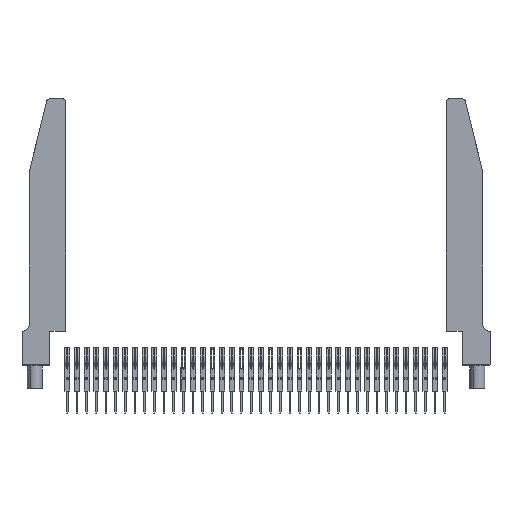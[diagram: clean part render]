
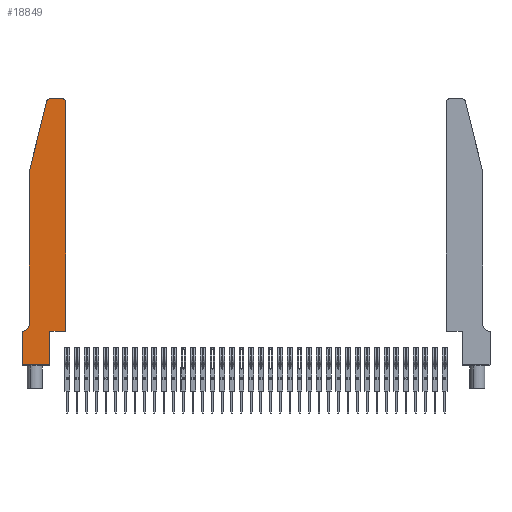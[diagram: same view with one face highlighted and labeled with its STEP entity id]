
A CAD part, top view. The second image highlights one B-rep face of the part: STEP entity #18849.
In plain terms, the highlighted planar face has unit normal (0, 0, 1).
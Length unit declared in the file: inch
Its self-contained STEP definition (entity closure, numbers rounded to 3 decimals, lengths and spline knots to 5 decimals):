
#72 = EDGE_CURVE ( 'NONE', #14185, #10593, #6628, .T. ) ;
#424 = ORIENTED_EDGE ( 'NONE', *, *, #72, .T. ) ;
#1006 = ORIENTED_EDGE ( 'NONE', *, *, #3949, .T. ) ;
#2183 = EDGE_CURVE ( 'NONE', #3761, #11347, #15558, .T. ) ;
#2339 = FACE_OUTER_BOUND ( 'NONE', #12901, .T. ) ;
#3177 = DIRECTION ( 'NONE',  ( -1., 0., 0. ) ) ;
#3275 = CARTESIAN_POINT ( 'NONE',  ( 0.2605, 2.75, 0.37 ) ) ;
#3415 = ORIENTED_EDGE ( 'NONE', *, *, #25045, .T. ) ;
#3742 = ORIENTED_EDGE ( 'NONE', *, *, #20649, .T. ) ;
#3761 = VERTEX_POINT ( 'NONE', #29488 ) ;
#3949 = EDGE_CURVE ( 'NONE', #28144, #14464, #5314, .T. ) ;
#4576 = VERTEX_POINT ( 'NONE', #20757 ) ;
#5207 = DIRECTION ( 'NONE',  ( -1., 0., 0. ) ) ;
#5306 = CARTESIAN_POINT ( 'NONE',  ( 0.2865, 0.35, 0.37 ) ) ;
#5314 = CIRCLE ( 'NONE', #13346, 0.07 ) ;
#5573 = VERTEX_POINT ( 'NONE', #18539 ) ;
#5587 = DIRECTION ( 'NONE',  ( -1., 0., 0. ) ) ;
#6424 = VECTOR ( 'NONE', #5587, 39.37008 ) ;
#6628 = LINE ( 'NONE', #18427, #9230 ) ;
#7030 = LINE ( 'NONE', #23628, #14231 ) ;
#7182 = VERTEX_POINT ( 'NONE', #7371 ) ;
#7371 = CARTESIAN_POINT ( 'NONE',  ( 0.25487, 2.72718, 0.37 ) ) ;
#7694 = DIRECTION ( 'NONE',  ( 0., 1., 0. ) ) ;
#8362 = CARTESIAN_POINT ( 'NONE',  ( 0.0055, 0.42, 0.37 ) ) ;
#8499 = DIRECTION ( 'NONE',  ( 0., -1., 0. ) ) ;
#8821 = CIRCLE ( 'NONE', #21907, 0.03 ) ;
#9230 = VECTOR ( 'NONE', #7694, 39.37008 ) ;
#9520 = VECTOR ( 'NONE', #32778, 39.37008 ) ;
#9580 = CARTESIAN_POINT ( 'NONE',  ( 0., 0.35, 0.37 ) ) ;
#10593 = VERTEX_POINT ( 'NONE', #5306 ) ;
#10608 = CARTESIAN_POINT ( 'NONE',  ( 0.4205, 2.75, 0.37 ) ) ;
#10736 = CARTESIAN_POINT ( 'NONE',  ( 0., 0.35, 0.37 ) ) ;
#10897 = ORIENTED_EDGE ( 'NONE', *, *, #23701, .T. ) ;
#11187 = EDGE_CURVE ( 'NONE', #7182, #29324, #7030, .T. ) ;
#11347 = VERTEX_POINT ( 'NONE', #10608 ) ;
#12293 = LINE ( 'NONE', #17648, #28172 ) ;
#12449 = VECTOR ( 'NONE', #31641, 39.37008 ) ;
#12901 = EDGE_LOOP ( 'NONE', ( #17440, #3742, #28590, #15875, #1006, #10897, #27812, #3415, #424, #24898, #13096, #30906 ) ) ;
#13096 = ORIENTED_EDGE ( 'NONE', *, *, #25732, .T. ) ;
#13346 = AXIS2_PLACEMENT_3D ( 'NONE', #8362, #14113, #3177 ) ;
#13997 = CARTESIAN_POINT ( 'NONE',  ( 0., 0., 0.37 ) ) ;
#14113 = DIRECTION ( 'NONE',  ( 0., 0., -1. ) ) ;
#14185 = VERTEX_POINT ( 'NONE', #18799 ) ;
#14231 = VECTOR ( 'NONE', #17410, 39.37008 ) ;
#14241 = VERTEX_POINT ( 'NONE', #21277 ) ;
#14464 = VERTEX_POINT ( 'NONE', #22531 ) ;
#15558 = CIRCLE ( 'NONE', #31065, 0.03 ) ;
#15684 = DIRECTION ( 'NONE',  ( 0., 0., 1. ) ) ;
#15696 = LINE ( 'NONE', #15880, #34674 ) ;
#15875 = ORIENTED_EDGE ( 'NONE', *, *, #19548, .T. ) ;
#15880 = CARTESIAN_POINT ( 'NONE',  ( 0.4505, 0.35, 0.37 ) ) ;
#16834 = LINE ( 'NONE', #13997, #9520 ) ;
#17410 = DIRECTION ( 'NONE',  ( -0.239, -0.971, 0. ) ) ;
#17440 = ORIENTED_EDGE ( 'NONE', *, *, #27198, .T. ) ;
#17648 = CARTESIAN_POINT ( 'NONE',  ( 0.0755, 2., 0.37 ) ) ;
#18427 = CARTESIAN_POINT ( 'NONE',  ( 0.2865, 0.35, 0.37 ) ) ;
#18539 = CARTESIAN_POINT ( 'NONE',  ( 0.284, 2.75, 0.37 ) ) ;
#18799 = CARTESIAN_POINT ( 'NONE',  ( 0.2865, 0., 0.37 ) ) ;
#18849 = ADVANCED_FACE ( 'NONE', ( #2339 ), #35235, .T. ) ;
#19548 = EDGE_CURVE ( 'NONE', #29324, #28144, #12293, .T. ) ;
#19966 = CARTESIAN_POINT ( 'NONE',  ( 0.4205, 2.72, 0.37 ) ) ;
#20649 = EDGE_CURVE ( 'NONE', #5573, #7182, #8821, .T. ) ;
#20757 = CARTESIAN_POINT ( 'NONE',  ( 0., 0., 0.37 ) ) ;
#21118 = LINE ( 'NONE', #29556, #29458 ) ;
#21277 = CARTESIAN_POINT ( 'NONE',  ( 0.4505, 0.35, 0.37 ) ) ;
#21907 = AXIS2_PLACEMENT_3D ( 'NONE', #23146, #15684, #34471 ) ;
#22531 = CARTESIAN_POINT ( 'NONE',  ( 0.0055, 0.35, 0.37 ) ) ;
#22934 = LINE ( 'NONE', #33198, #24058 ) ;
#23146 = CARTESIAN_POINT ( 'NONE',  ( 0.284, 2.72, 0.37 ) ) ;
#23316 = DIRECTION ( 'NONE',  ( 1., 0., 0. ) ) ;
#23628 = CARTESIAN_POINT ( 'NONE',  ( 0.0755, 2., 0.37 ) ) ;
#23701 = EDGE_CURVE ( 'NONE', #14464, #28133, #21118, .T. ) ;
#24058 = VECTOR ( 'NONE', #8499, 39.37008 ) ;
#24898 = ORIENTED_EDGE ( 'NONE', *, *, #33653, .T. ) ;
#25045 = EDGE_CURVE ( 'NONE', #4576, #14185, #16834, .T. ) ;
#25732 = EDGE_CURVE ( 'NONE', #14241, #3761, #34319, .T. ) ;
#26169 = CARTESIAN_POINT ( 'NONE',  ( 0.0755, 0.42, 0.37 ) ) ;
#26222 = CARTESIAN_POINT ( 'NONE',  ( 0.0755, 2., 0.37 ) ) ;
#26921 = DIRECTION ( 'NONE',  ( 1., 0., 0. ) ) ;
#27171 = DIRECTION ( 'NONE',  ( 0., 0., 1. ) ) ;
#27198 = EDGE_CURVE ( 'NONE', #11347, #5573, #27751, .T. ) ;
#27751 = LINE ( 'NONE', #3275, #6424 ) ;
#27812 = ORIENTED_EDGE ( 'NONE', *, *, #27952, .T. ) ;
#27952 = EDGE_CURVE ( 'NONE', #28133, #4576, #22934, .T. ) ;
#28133 = VERTEX_POINT ( 'NONE', #9580 ) ;
#28144 = VERTEX_POINT ( 'NONE', #26169 ) ;
#28172 = VECTOR ( 'NONE', #33938, 39.37008 ) ;
#28555 = DIRECTION ( 'NONE',  ( 0., 0., 1. ) ) ;
#28590 = ORIENTED_EDGE ( 'NONE', *, *, #11187, .T. ) ;
#29324 = VERTEX_POINT ( 'NONE', #26222 ) ;
#29458 = VECTOR ( 'NONE', #5207, 39.37008 ) ;
#29488 = CARTESIAN_POINT ( 'NONE',  ( 0.4505, 2.72, 0.37 ) ) ;
#29556 = CARTESIAN_POINT ( 'NONE',  ( 0.0755, 0.35, 0.37 ) ) ;
#29838 = AXIS2_PLACEMENT_3D ( 'NONE', #10736, #27171, #32567 ) ;
#30906 = ORIENTED_EDGE ( 'NONE', *, *, #2183, .T. ) ;
#31065 = AXIS2_PLACEMENT_3D ( 'NONE', #19966, #28555, #23316 ) ;
#31641 = DIRECTION ( 'NONE',  ( 0., 1., 0. ) ) ;
#32567 = DIRECTION ( 'NONE',  ( 1., 0., 0. ) ) ;
#32778 = DIRECTION ( 'NONE',  ( 1., 0., 0. ) ) ;
#33198 = CARTESIAN_POINT ( 'NONE',  ( 0., 0., 0.37 ) ) ;
#33653 = EDGE_CURVE ( 'NONE', #10593, #14241, #15696, .T. ) ;
#33938 = DIRECTION ( 'NONE',  ( 0., -1., 0. ) ) ;
#34319 = LINE ( 'NONE', #34493, #12449 ) ;
#34471 = DIRECTION ( 'NONE',  ( 1., 0., 0. ) ) ;
#34493 = CARTESIAN_POINT ( 'NONE',  ( 0.4505, 0.35, 0.37 ) ) ;
#34674 = VECTOR ( 'NONE', #26921, 39.37008 ) ;
#35235 = PLANE ( 'NONE',  #29838 ) ;
